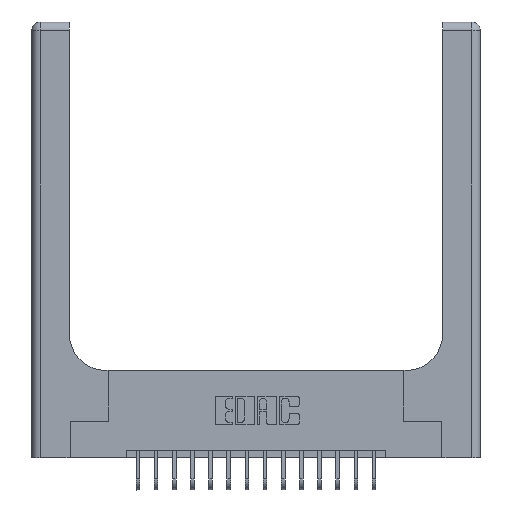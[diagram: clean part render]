
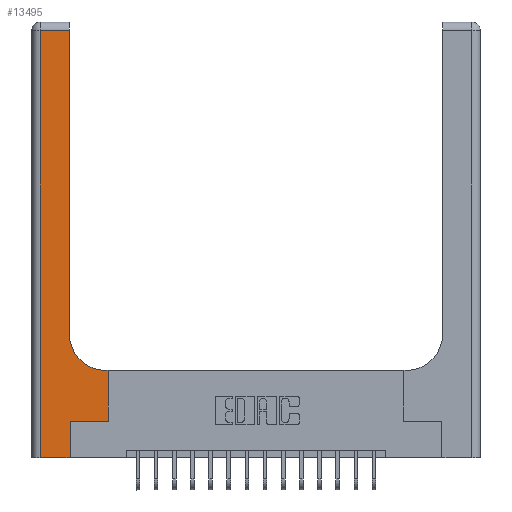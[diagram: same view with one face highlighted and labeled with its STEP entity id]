
A CAD part, top view. The second image highlights one B-rep face of the part: STEP entity #13495.
In plain terms, the highlighted planar face has unit normal (0, 0, 1).
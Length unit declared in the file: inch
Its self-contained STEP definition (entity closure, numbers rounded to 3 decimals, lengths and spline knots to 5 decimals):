
#353 = CARTESIAN_POINT ( 'NONE',  ( 0., 2.94, 0.37 ) ) ;
#382 = FACE_OUTER_BOUND ( 'NONE', #9643, .T. ) ;
#1362 = LINE ( 'NONE', #4004, #17229 ) ;
#1434 = EDGE_CURVE ( 'NONE', #13558, #9822, #13058, .T. ) ;
#1934 = ORIENTED_EDGE ( 'NONE', *, *, #7226, .T. ) ;
#2232 = VECTOR ( 'NONE', #17118, 39.37008 ) ;
#2487 = LINE ( 'NONE', #11538, #16199 ) ;
#2577 = LINE ( 'NONE', #16109, #4237 ) ;
#2699 = AXIS2_PLACEMENT_3D ( 'NONE', #3047, #6279, #10921 ) ;
#2936 = VECTOR ( 'NONE', #19873, 39.37008 ) ;
#3047 = CARTESIAN_POINT ( 'NONE',  ( 0., 3., 0.37 ) ) ;
#3260 = PLANE ( 'NONE',  #2699 ) ;
#3572 = CARTESIAN_POINT ( 'NONE',  ( 0.06, 0., 0.37 ) ) ;
#3758 = EDGE_CURVE ( 'NONE', #12756, #12998, #6249, .T. ) ;
#3928 = DIRECTION ( 'NONE',  ( 0., 1., 0. ) ) ;
#3962 = LINE ( 'NONE', #11454, #15053 ) ;
#4004 = CARTESIAN_POINT ( 'NONE',  ( 0.06, 3., 0.37 ) ) ;
#4237 = VECTOR ( 'NONE', #3928, 39.37008 ) ;
#4588 = ORIENTED_EDGE ( 'NONE', *, *, #13174, .T. ) ;
#5137 = CARTESIAN_POINT ( 'NONE',  ( 0.51, 0.6, 0.37 ) ) ;
#5209 = AXIS2_PLACEMENT_3D ( 'NONE', #7365, #7108, #16466 ) ;
#5536 = DIRECTION ( 'NONE',  ( 1., 0., 0. ) ) ;
#5579 = CARTESIAN_POINT ( 'NONE',  ( 0.265, 0., 0.37 ) ) ;
#5726 = VERTEX_POINT ( 'NONE', #6546 ) ;
#5762 = VECTOR ( 'NONE', #10815, 39.37008 ) ;
#5820 = ORIENTED_EDGE ( 'NONE', *, *, #15003, .T. ) ;
#6126 = ORIENTED_EDGE ( 'NONE', *, *, #10366, .T. ) ;
#6249 = LINE ( 'NONE', #9421, #5762 ) ;
#6279 = DIRECTION ( 'NONE',  ( 0., 0., -1. ) ) ;
#6360 = CARTESIAN_POINT ( 'NONE',  ( 0.26, 2.94, 0.37 ) ) ;
#6546 = CARTESIAN_POINT ( 'NONE',  ( 0.265, 0.25, 0.37 ) ) ;
#6578 = LINE ( 'NONE', #353, #9728 ) ;
#6895 = DIRECTION ( 'NONE',  ( 0., -1., 0. ) ) ;
#7108 = DIRECTION ( 'NONE',  ( 0., 0., -1. ) ) ;
#7226 = EDGE_CURVE ( 'NONE', #9127, #12756, #2577, .T. ) ;
#7365 = CARTESIAN_POINT ( 'NONE',  ( 0.51, 0.85, 0.37 ) ) ;
#7628 = CARTESIAN_POINT ( 'NONE',  ( 0., 0., 0.37 ) ) ;
#8297 = ORIENTED_EDGE ( 'NONE', *, *, #3758, .T. ) ;
#8650 = ORIENTED_EDGE ( 'NONE', *, *, #13701, .T. ) ;
#9101 = CARTESIAN_POINT ( 'NONE',  ( 0.528, 0.6, 0.37 ) ) ;
#9127 = VERTEX_POINT ( 'NONE', #18368 ) ;
#9207 = CARTESIAN_POINT ( 'NONE',  ( 0.26, 3., 0.37 ) ) ;
#9421 = CARTESIAN_POINT ( 'NONE',  ( 0.26, 0.6, 0.37 ) ) ;
#9643 = EDGE_LOOP ( 'NONE', ( #16222, #18182, #4588, #13522, #8650, #5820, #1934, #8297, #6126 ) ) ;
#9728 = VECTOR ( 'NONE', #17481, 39.37008 ) ;
#9822 = VERTEX_POINT ( 'NONE', #6360 ) ;
#9897 = VERTEX_POINT ( 'NONE', #3572 ) ;
#10268 = VERTEX_POINT ( 'NONE', #11431 ) ;
#10366 = EDGE_CURVE ( 'NONE', #12998, #13558, #14972, .T. ) ;
#10439 = EDGE_CURVE ( 'NONE', #9897, #11439, #18794, .T. ) ;
#10815 = DIRECTION ( 'NONE',  ( -1., 0., 0. ) ) ;
#10921 = DIRECTION ( 'NONE',  ( -1., 0., 0. ) ) ;
#11431 = CARTESIAN_POINT ( 'NONE',  ( 0.06, 2.94, 0.37 ) ) ;
#11439 = VERTEX_POINT ( 'NONE', #5579 ) ;
#11454 = CARTESIAN_POINT ( 'NONE',  ( 0.265, 0., 0.37 ) ) ;
#11538 = CARTESIAN_POINT ( 'NONE',  ( 0.265, 0.25, 0.37 ) ) ;
#12756 = VERTEX_POINT ( 'NONE', #9101 ) ;
#12998 = VERTEX_POINT ( 'NONE', #5137 ) ;
#13058 = LINE ( 'NONE', #9207, #2232 ) ;
#13147 = DIRECTION ( 'NONE',  ( 0., 1., 0. ) ) ;
#13174 = EDGE_CURVE ( 'NONE', #10268, #9897, #1362, .T. ) ;
#13495 = ADVANCED_FACE ( 'NONE', ( #382 ), #3260, .F. ) ;
#13522 = ORIENTED_EDGE ( 'NONE', *, *, #10439, .T. ) ;
#13558 = VERTEX_POINT ( 'NONE', #17161 ) ;
#13701 = EDGE_CURVE ( 'NONE', #11439, #5726, #3962, .T. ) ;
#14331 = EDGE_CURVE ( 'NONE', #9822, #10268, #6578, .T. ) ;
#14972 = CIRCLE ( 'NONE', #5209, 0.25 ) ;
#15003 = EDGE_CURVE ( 'NONE', #5726, #9127, #2487, .T. ) ;
#15053 = VECTOR ( 'NONE', #13147, 39.37008 ) ;
#16109 = CARTESIAN_POINT ( 'NONE',  ( 0.528, 0.25, 0.37 ) ) ;
#16199 = VECTOR ( 'NONE', #5536, 39.37008 ) ;
#16222 = ORIENTED_EDGE ( 'NONE', *, *, #1434, .T. ) ;
#16466 = DIRECTION ( 'NONE',  ( 1., 0., 0. ) ) ;
#17118 = DIRECTION ( 'NONE',  ( 0., 1., 0. ) ) ;
#17161 = CARTESIAN_POINT ( 'NONE',  ( 0.26, 0.85, 0.37 ) ) ;
#17229 = VECTOR ( 'NONE', #6895, 39.37008 ) ;
#17481 = DIRECTION ( 'NONE',  ( -1., 0., 0. ) ) ;
#18182 = ORIENTED_EDGE ( 'NONE', *, *, #14331, .T. ) ;
#18368 = CARTESIAN_POINT ( 'NONE',  ( 0.528, 0.25, 0.37 ) ) ;
#18794 = LINE ( 'NONE', #7628, #2936 ) ;
#19873 = DIRECTION ( 'NONE',  ( 1., 0., 0. ) ) ;
